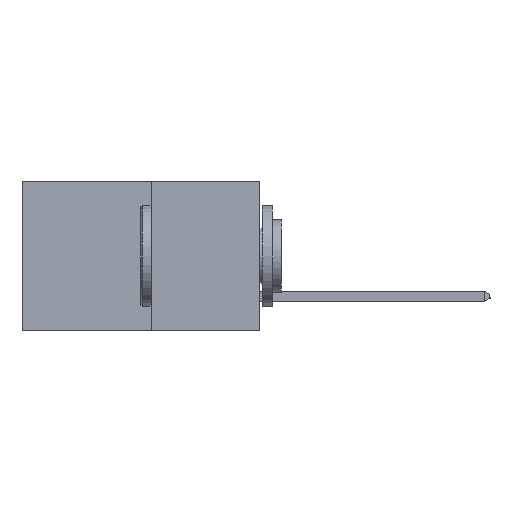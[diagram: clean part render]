
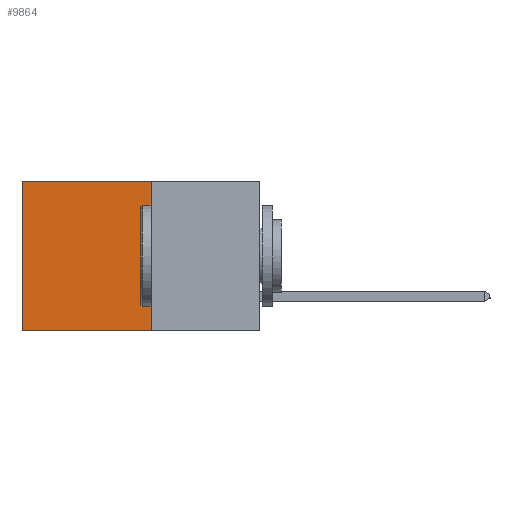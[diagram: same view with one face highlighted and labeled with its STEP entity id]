
A CAD part, left-side view. The second image highlights one B-rep face of the part: STEP entity #9864.
In plain terms, the highlighted planar face has unit normal (-1, 0, 0).
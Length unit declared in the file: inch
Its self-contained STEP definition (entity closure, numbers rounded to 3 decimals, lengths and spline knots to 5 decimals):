
#385 = VECTOR ( 'NONE', #13656, 39.37008 ) ;
#878 = EDGE_LOOP ( 'NONE', ( #4224, #12441, #1222, #3442 ) ) ;
#1222 = ORIENTED_EDGE ( 'NONE', *, *, #3629, .F. ) ;
#1676 = EDGE_CURVE ( 'NONE', #12367, #11702, #7667, .T. ) ;
#1945 = CARTESIAN_POINT ( 'NONE',  ( 0.277, 0.59, 0. ) ) ;
#2007 = DIRECTION ( 'NONE',  ( 0., 0., -1. ) ) ;
#2050 = CARTESIAN_POINT ( 'NONE',  ( 0.277, 0.59, -0.37 ) ) ;
#2425 = CARTESIAN_POINT ( 'NONE',  ( 0.277, 0.27, -0.37 ) ) ;
#2517 = VERTEX_POINT ( 'NONE', #14293 ) ;
#2985 = LINE ( 'NONE', #14360, #15503 ) ;
#3115 = CARTESIAN_POINT ( 'NONE',  ( 0.277, 0.59, -0.37 ) ) ;
#3442 = ORIENTED_EDGE ( 'NONE', *, *, #9059, .T. ) ;
#3629 = EDGE_CURVE ( 'NONE', #8830, #2517, #4466, .T. ) ;
#3657 = AXIS2_PLACEMENT_3D ( 'NONE', #5213, #6446, #14910 ) ;
#3963 = PLANE ( 'NONE',  #3657 ) ;
#3983 = EDGE_CURVE ( 'NONE', #2517, #11702, #11750, .T. ) ;
#4224 = ORIENTED_EDGE ( 'NONE', *, *, #1676, .T. ) ;
#4466 = LINE ( 'NONE', #2425, #10664 ) ;
#5213 = CARTESIAN_POINT ( 'NONE',  ( 0.277, 0.27, -0.37 ) ) ;
#6446 = DIRECTION ( 'NONE',  ( 1., 0., 0. ) ) ;
#7667 = LINE ( 'NONE', #2050, #385 ) ;
#8830 = VERTEX_POINT ( 'NONE', #13992 ) ;
#9059 = EDGE_CURVE ( 'NONE', #8830, #12367, #2985, .T. ) ;
#9192 = CARTESIAN_POINT ( 'NONE',  ( 0.277, 0.27, -0.37 ) ) ;
#9318 = DIRECTION ( 'NONE',  ( 0., 1., 0. ) ) ;
#9864 = ADVANCED_FACE ( 'NONE', ( #14217 ), #3963, .F. ) ;
#10664 = VECTOR ( 'NONE', #2007, 39.37008 ) ;
#11076 = DIRECTION ( 'NONE',  ( 0., 1., 0. ) ) ;
#11702 = VERTEX_POINT ( 'NONE', #3115 ) ;
#11750 = LINE ( 'NONE', #9192, #14532 ) ;
#12367 = VERTEX_POINT ( 'NONE', #1945 ) ;
#12441 = ORIENTED_EDGE ( 'NONE', *, *, #3983, .F. ) ;
#13656 = DIRECTION ( 'NONE',  ( 0., 0., -1. ) ) ;
#13992 = CARTESIAN_POINT ( 'NONE',  ( 0.277, 0.27, 0. ) ) ;
#14217 = FACE_OUTER_BOUND ( 'NONE', #878, .T. ) ;
#14293 = CARTESIAN_POINT ( 'NONE',  ( 0.277, 0.27, -0.37 ) ) ;
#14360 = CARTESIAN_POINT ( 'NONE',  ( 0.277, 0.27, 0. ) ) ;
#14532 = VECTOR ( 'NONE', #9318, 39.37008 ) ;
#14910 = DIRECTION ( 'NONE',  ( 0., 0., -1. ) ) ;
#15503 = VECTOR ( 'NONE', #11076, 39.37008 ) ;
